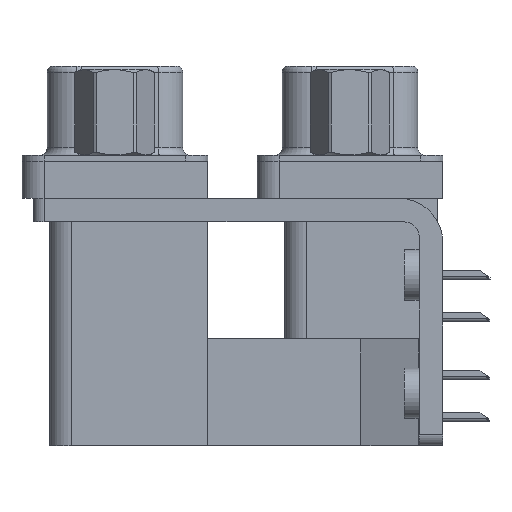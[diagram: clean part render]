
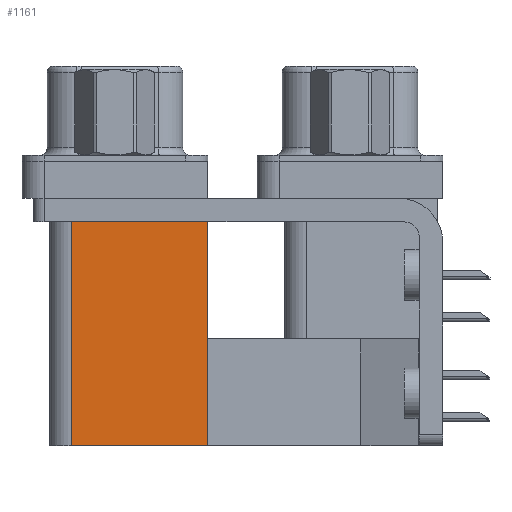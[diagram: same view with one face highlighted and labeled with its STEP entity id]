
A CAD part, left-side view. The second image highlights one B-rep face of the part: STEP entity #1161.
In plain terms, the highlighted planar face has unit normal (-1, 0, 0).
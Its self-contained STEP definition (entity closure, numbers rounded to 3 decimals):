
#246 = LINE ( 'NONE', #20653, #15920 ) ;
#1161 = ADVANCED_FACE ( 'NONE', ( #21620 ), #8908, .F. ) ;
#1471 = CARTESIAN_POINT ( 'NONE',  ( 3.79, 9.6, -19.2 ) ) ;
#1860 = EDGE_CURVE ( 'NONE', #3522, #2607, #12559, .T. ) ;
#2607 = VERTEX_POINT ( 'NONE', #2905 ) ;
#2905 = CARTESIAN_POINT ( 'NONE',  ( 3.79, 18.8, -2.5 ) ) ;
#3522 = VERTEX_POINT ( 'NONE', #23543 ) ;
#3568 = VERTEX_POINT ( 'NONE', #26857 ) ;
#4690 = LINE ( 'NONE', #25402, #19923 ) ;
#7927 = DIRECTION ( 'NONE',  ( 0., 0., 1. ) ) ;
#8332 = ORIENTED_EDGE ( 'NONE', *, *, #1860, .T. ) ;
#8396 = ORIENTED_EDGE ( 'NONE', *, *, #10416, .F. ) ;
#8908 = PLANE ( 'NONE',  #18559 ) ;
#10416 = EDGE_CURVE ( 'NONE', #3568, #2607, #246, .T. ) ;
#12559 = LINE ( 'NONE', #17572, #18971 ) ;
#12890 = VERTEX_POINT ( 'NONE', #1471 ) ;
#14917 = DIRECTION ( 'NONE',  ( 0., 1., 0. ) ) ;
#15320 = EDGE_CURVE ( 'NONE', #12890, #3568, #4690, .T. ) ;
#15920 = VECTOR ( 'NONE', #7927, 1000. ) ;
#17572 = CARTESIAN_POINT ( 'NONE',  ( 3.79, 9.6, -2.5 ) ) ;
#18559 = AXIS2_PLACEMENT_3D ( 'NONE', #29611, #26769, #24762 ) ;
#18971 = VECTOR ( 'NONE', #19913, 1000. ) ;
#19913 = DIRECTION ( 'NONE',  ( 0., 1., 0. ) ) ;
#19923 = VECTOR ( 'NONE', #14917, 1000. ) ;
#20653 = CARTESIAN_POINT ( 'NONE',  ( 3.79, 18.8, -19.2 ) ) ;
#21620 = FACE_OUTER_BOUND ( 'NONE', #22278, .T. ) ;
#21853 = EDGE_CURVE ( 'NONE', #12890, #3522, #22957, .T. ) ;
#22278 = EDGE_LOOP ( 'NONE', ( #8332, #8396, #29082, #29228 ) ) ;
#22636 = CARTESIAN_POINT ( 'NONE',  ( 3.79, 9.6, -19.2 ) ) ;
#22957 = LINE ( 'NONE', #22636, #31956 ) ;
#23543 = CARTESIAN_POINT ( 'NONE',  ( 3.79, 9.6, -2.5 ) ) ;
#24762 = DIRECTION ( 'NONE',  ( 0., 0., -1. ) ) ;
#25402 = CARTESIAN_POINT ( 'NONE',  ( 3.79, 9.6, -19.2 ) ) ;
#26769 = DIRECTION ( 'NONE',  ( 1., 0., 0. ) ) ;
#26857 = CARTESIAN_POINT ( 'NONE',  ( 3.79, 18.8, -19.2 ) ) ;
#29082 = ORIENTED_EDGE ( 'NONE', *, *, #15320, .F. ) ;
#29228 = ORIENTED_EDGE ( 'NONE', *, *, #21853, .T. ) ;
#29611 = CARTESIAN_POINT ( 'NONE',  ( 3.79, 9.6, -19.2 ) ) ;
#31956 = VECTOR ( 'NONE', #32821, 1000. ) ;
#32821 = DIRECTION ( 'NONE',  ( 0., 0., 1. ) ) ;
